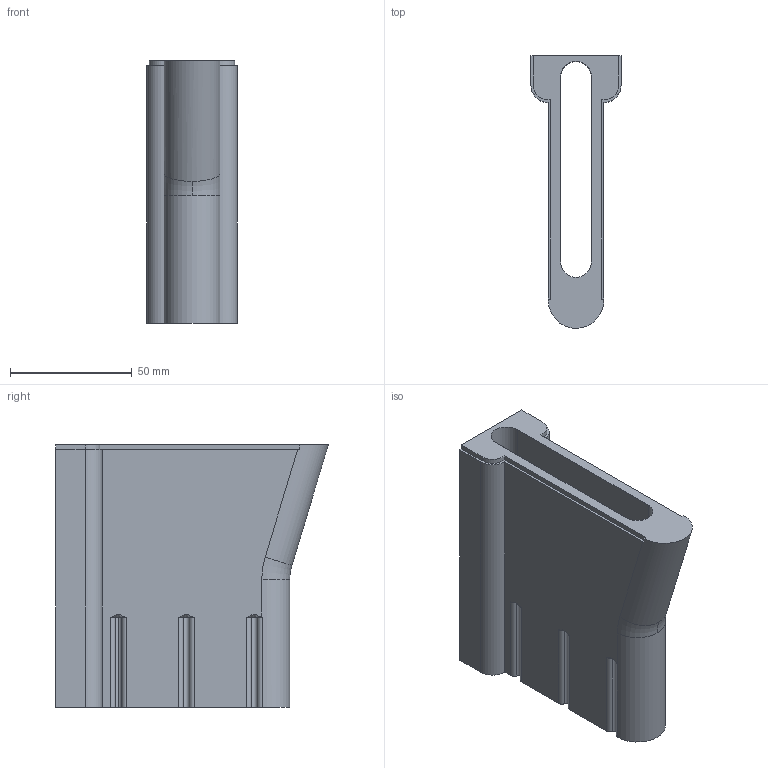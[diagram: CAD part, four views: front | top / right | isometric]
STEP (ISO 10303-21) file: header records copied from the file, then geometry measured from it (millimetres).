
FILE_DESCRIPTION (( 'STEP AP214' ), '1' );
FILE_NAME ('Charon_V3_Rifle_2.STEP', '2013-09-01T16:54:58', ( 'Asher' ), ( '' ), 'SwSTEP 2.0', 'SolidWorks 2013', '' );
FILE_SCHEMA (( 'AUTOMOTIVE_DESIGN' ));
Length unit declared in the file: millimetre
Products named in the file (1): Charon_V3_Rifle_2
Bounding box: 37.13 x 112.17 x 108 mm (x, y, z)
Volume: 149059 mm3; surface area: 52566.5 mm2
Topology: 1 solids, 1 shells, 107 faces, 324 edges, 215 vertices
Faces by surface type: cylinder 32, sphere 28, plane 23, cone 22, torus 2
Entity records: 3445 total; most frequent: CARTESIAN_POINT 679, DIRECTION 614, ORIENTED_EDGE 544, EDGE_CURVE 272, AXIS2_PLACEMENT_3D 254, VERTEX_POINT 191, CIRCLE 146, EDGE_LOOP 133
